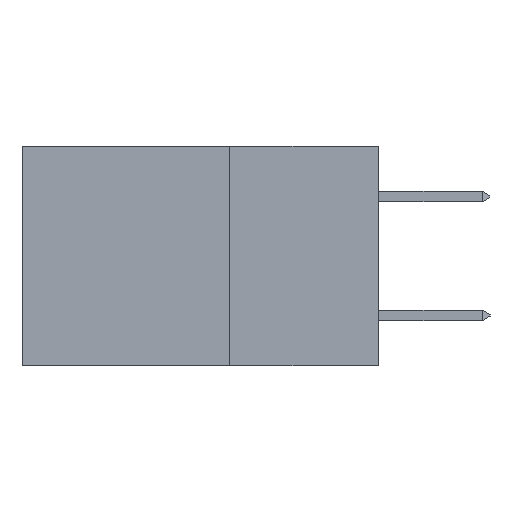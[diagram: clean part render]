
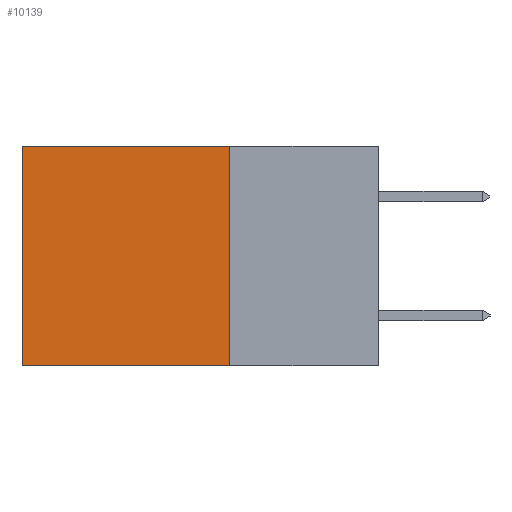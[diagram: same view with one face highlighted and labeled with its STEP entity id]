
A CAD part, left-side view. The second image highlights one B-rep face of the part: STEP entity #10139.
In plain terms, the highlighted planar face has unit normal (-1, 0, 0).
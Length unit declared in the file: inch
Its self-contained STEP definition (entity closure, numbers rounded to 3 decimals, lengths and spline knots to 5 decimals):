
#26 = CARTESIAN_POINT ( 'NONE',  ( 0.2615, 0.25, 0. ) ) ;
#643 = VECTOR ( 'NONE', #2240, 39.37008 ) ;
#782 = AXIS2_PLACEMENT_3D ( 'NONE', #2514, #3558, #10859 ) ;
#970 = LINE ( 'NONE', #7458, #643 ) ;
#1335 = VERTEX_POINT ( 'NONE', #5669 ) ;
#1441 = ORIENTED_EDGE ( 'NONE', *, *, #7077, .T. ) ;
#1510 = EDGE_CURVE ( 'NONE', #10313, #1335, #10780, .T. ) ;
#2240 = DIRECTION ( 'NONE',  ( 0., 0., -1. ) ) ;
#2514 = CARTESIAN_POINT ( 'NONE',  ( 0.2615, 0.25, -0.37 ) ) ;
#2759 = VECTOR ( 'NONE', #4403, 39.37008 ) ;
#3192 = FACE_OUTER_BOUND ( 'NONE', #10035, .T. ) ;
#3281 = DIRECTION ( 'NONE',  ( 0., 1., 0. ) ) ;
#3558 = DIRECTION ( 'NONE',  ( 1., 0., 0. ) ) ;
#4403 = DIRECTION ( 'NONE',  ( 0., 0., -1. ) ) ;
#5461 = CARTESIAN_POINT ( 'NONE',  ( 0.2615, 0.6, -0.37 ) ) ;
#5523 = VERTEX_POINT ( 'NONE', #8074 ) ;
#5669 = CARTESIAN_POINT ( 'NONE',  ( 0.2615, 0.6, 0. ) ) ;
#6522 = ORIENTED_EDGE ( 'NONE', *, *, #7033, .F. ) ;
#6965 = CARTESIAN_POINT ( 'NONE',  ( 0.2615, 0.25, 0. ) ) ;
#7020 = EDGE_CURVE ( 'NONE', #10313, #12448, #970, .T. ) ;
#7033 = EDGE_CURVE ( 'NONE', #12448, #5523, #11735, .T. ) ;
#7077 = EDGE_CURVE ( 'NONE', #1335, #5523, #8328, .T. ) ;
#7458 = CARTESIAN_POINT ( 'NONE',  ( 0.2615, 0.25, -0.37 ) ) ;
#8021 = VECTOR ( 'NONE', #12650, 39.37008 ) ;
#8058 = ORIENTED_EDGE ( 'NONE', *, *, #1510, .T. ) ;
#8074 = CARTESIAN_POINT ( 'NONE',  ( 0.2615, 0.6, -0.37 ) ) ;
#8328 = LINE ( 'NONE', #5461, #2759 ) ;
#8771 = PLANE ( 'NONE',  #782 ) ;
#10035 = EDGE_LOOP ( 'NONE', ( #1441, #6522, #10792, #8058 ) ) ;
#10139 = ADVANCED_FACE ( 'NONE', ( #3192 ), #8771, .F. ) ;
#10313 = VERTEX_POINT ( 'NONE', #6965 ) ;
#10780 = LINE ( 'NONE', #26, #8021 ) ;
#10792 = ORIENTED_EDGE ( 'NONE', *, *, #7020, .F. ) ;
#10859 = DIRECTION ( 'NONE',  ( 0., 0., -1. ) ) ;
#10978 = CARTESIAN_POINT ( 'NONE',  ( 0.2615, 0.25, -0.37 ) ) ;
#11418 = VECTOR ( 'NONE', #3281, 39.37008 ) ;
#11621 = CARTESIAN_POINT ( 'NONE',  ( 0.2615, 0.25, -0.37 ) ) ;
#11735 = LINE ( 'NONE', #11621, #11418 ) ;
#12448 = VERTEX_POINT ( 'NONE', #10978 ) ;
#12650 = DIRECTION ( 'NONE',  ( 0., 1., 0. ) ) ;
